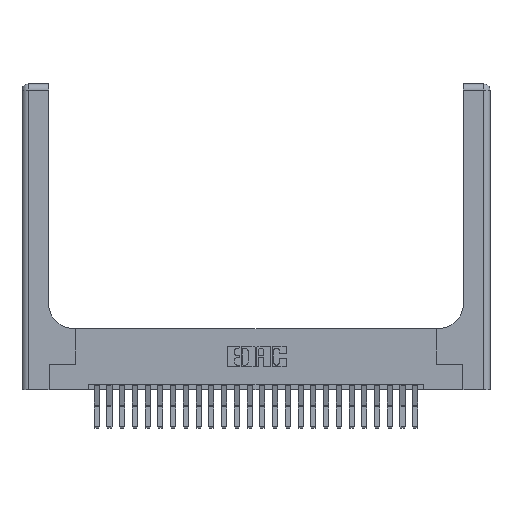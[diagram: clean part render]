
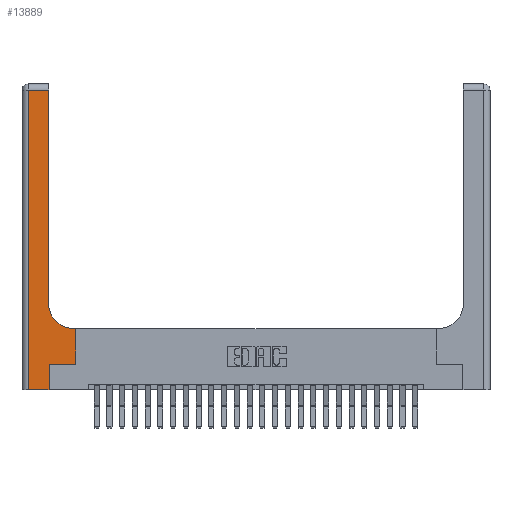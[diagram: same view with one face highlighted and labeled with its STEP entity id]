
A CAD part, top view. The second image highlights one B-rep face of the part: STEP entity #13889.
In plain terms, the highlighted planar face has unit normal (0, 0, 1).
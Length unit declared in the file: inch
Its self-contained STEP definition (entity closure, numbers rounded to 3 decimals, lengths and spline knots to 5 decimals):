
#484 = CARTESIAN_POINT ( 'NONE',  ( 0.51, 0.6, 0.37 ) ) ;
#2607 = VERTEX_POINT ( 'NONE', #21741 ) ;
#2796 = EDGE_CURVE ( 'NONE', #6051, #24206, #3019, .T. ) ;
#3019 = LINE ( 'NONE', #10699, #13411 ) ;
#3045 = VERTEX_POINT ( 'NONE', #20966 ) ;
#3153 = EDGE_CURVE ( 'NONE', #7943, #16102, #13583, .T. ) ;
#3191 = LINE ( 'NONE', #21906, #19430 ) ;
#3268 = PLANE ( 'NONE',  #17568 ) ;
#3340 = CARTESIAN_POINT ( 'NONE',  ( 0.06, 2.94, 0.37 ) ) ;
#3847 = VECTOR ( 'NONE', #20916, 39.37008 ) ;
#4181 = ORIENTED_EDGE ( 'NONE', *, *, #2796, .T. ) ;
#4547 = VERTEX_POINT ( 'NONE', #23224 ) ;
#4980 = VECTOR ( 'NONE', #13824, 39.37008 ) ;
#4985 = VECTOR ( 'NONE', #20823, 39.37008 ) ;
#5691 = EDGE_CURVE ( 'NONE', #17045, #9990, #9765, .T. ) ;
#5738 = CARTESIAN_POINT ( 'NONE',  ( 0.26, 0.6, 0.37 ) ) ;
#5907 = DIRECTION ( 'NONE',  ( -1., 0., 0. ) ) ;
#5972 = EDGE_CURVE ( 'NONE', #9990, #2607, #17877, .T. ) ;
#6051 = VERTEX_POINT ( 'NONE', #3340 ) ;
#6057 = DIRECTION ( 'NONE',  ( 0., 1., 0. ) ) ;
#6106 = EDGE_CURVE ( 'NONE', #16102, #17045, #7473, .T. ) ;
#6836 = ORIENTED_EDGE ( 'NONE', *, *, #21724, .T. ) ;
#7473 = LINE ( 'NONE', #18917, #3847 ) ;
#7943 = VERTEX_POINT ( 'NONE', #23792 ) ;
#8121 = ORIENTED_EDGE ( 'NONE', *, *, #19393, .T. ) ;
#8127 = ORIENTED_EDGE ( 'NONE', *, *, #21030, .T. ) ;
#8785 = FACE_OUTER_BOUND ( 'NONE', #21935, .T. ) ;
#8973 = CARTESIAN_POINT ( 'NONE',  ( 0.528, 0.25, 0.37 ) ) ;
#9025 = VECTOR ( 'NONE', #12688, 39.37008 ) ;
#9040 = DIRECTION ( 'NONE',  ( -1., 0., 0. ) ) ;
#9256 = CARTESIAN_POINT ( 'NONE',  ( 0.528, 0.6, 0.37 ) ) ;
#9765 = LINE ( 'NONE', #5738, #4985 ) ;
#9968 = ORIENTED_EDGE ( 'NONE', *, *, #5972, .T. ) ;
#9990 = VERTEX_POINT ( 'NONE', #484 ) ;
#10212 = LINE ( 'NONE', #17760, #21886 ) ;
#10324 = CARTESIAN_POINT ( 'NONE',  ( 0.06, 0., 0.37 ) ) ;
#10699 = CARTESIAN_POINT ( 'NONE',  ( 0.06, 3., 0.37 ) ) ;
#11335 = LINE ( 'NONE', #24800, #16090 ) ;
#12688 = DIRECTION ( 'NONE',  ( 1., 0., 0. ) ) ;
#13411 = VECTOR ( 'NONE', #20350, 39.37008 ) ;
#13583 = LINE ( 'NONE', #13706, #4980 ) ;
#13706 = CARTESIAN_POINT ( 'NONE',  ( 0.265, 0.25, 0.37 ) ) ;
#13824 = DIRECTION ( 'NONE',  ( 1., 0., 0. ) ) ;
#13889 = ADVANCED_FACE ( 'NONE', ( #8785 ), #3268, .F. ) ;
#14347 = ORIENTED_EDGE ( 'NONE', *, *, #3153, .T. ) ;
#14576 = CARTESIAN_POINT ( 'NONE',  ( 0., 0., 0.37 ) ) ;
#14847 = EDGE_CURVE ( 'NONE', #3045, #6051, #11335, .T. ) ;
#16090 = VECTOR ( 'NONE', #5907, 39.37008 ) ;
#16102 = VERTEX_POINT ( 'NONE', #8973 ) ;
#16276 = DIRECTION ( 'NONE',  ( 0., 1., 0. ) ) ;
#16551 = ORIENTED_EDGE ( 'NONE', *, *, #5691, .T. ) ;
#16680 = DIRECTION ( 'NONE',  ( 1., 0., 0. ) ) ;
#17045 = VERTEX_POINT ( 'NONE', #9256 ) ;
#17568 = AXIS2_PLACEMENT_3D ( 'NONE', #18598, #24390, #9040 ) ;
#17760 = CARTESIAN_POINT ( 'NONE',  ( 0.26, 3., 0.37 ) ) ;
#17877 = CIRCLE ( 'NONE', #21072, 0.25 ) ;
#18091 = LINE ( 'NONE', #14576, #9025 ) ;
#18181 = CARTESIAN_POINT ( 'NONE',  ( 0.51, 0.85, 0.37 ) ) ;
#18598 = CARTESIAN_POINT ( 'NONE',  ( 0., 3., 0.37 ) ) ;
#18917 = CARTESIAN_POINT ( 'NONE',  ( 0.528, 0.25, 0.37 ) ) ;
#19393 = EDGE_CURVE ( 'NONE', #4547, #7943, #3191, .T. ) ;
#19430 = VECTOR ( 'NONE', #16276, 39.37008 ) ;
#20350 = DIRECTION ( 'NONE',  ( 0., -1., 0. ) ) ;
#20823 = DIRECTION ( 'NONE',  ( -1., 0., 0. ) ) ;
#20916 = DIRECTION ( 'NONE',  ( 0., 1., 0. ) ) ;
#20966 = CARTESIAN_POINT ( 'NONE',  ( 0.26, 2.94, 0.37 ) ) ;
#21030 = EDGE_CURVE ( 'NONE', #2607, #3045, #10212, .T. ) ;
#21072 = AXIS2_PLACEMENT_3D ( 'NONE', #18181, #22439, #16680 ) ;
#21724 = EDGE_CURVE ( 'NONE', #24206, #4547, #18091, .T. ) ;
#21741 = CARTESIAN_POINT ( 'NONE',  ( 0.26, 0.85, 0.37 ) ) ;
#21886 = VECTOR ( 'NONE', #6057, 39.37008 ) ;
#21906 = CARTESIAN_POINT ( 'NONE',  ( 0.265, 0., 0.37 ) ) ;
#21935 = EDGE_LOOP ( 'NONE', ( #8127, #23402, #4181, #6836, #8121, #14347, #22312, #16551, #9968 ) ) ;
#22312 = ORIENTED_EDGE ( 'NONE', *, *, #6106, .T. ) ;
#22439 = DIRECTION ( 'NONE',  ( 0., 0., -1. ) ) ;
#23224 = CARTESIAN_POINT ( 'NONE',  ( 0.265, 0., 0.37 ) ) ;
#23402 = ORIENTED_EDGE ( 'NONE', *, *, #14847, .T. ) ;
#23792 = CARTESIAN_POINT ( 'NONE',  ( 0.265, 0.25, 0.37 ) ) ;
#24206 = VERTEX_POINT ( 'NONE', #10324 ) ;
#24390 = DIRECTION ( 'NONE',  ( 0., 0., -1. ) ) ;
#24800 = CARTESIAN_POINT ( 'NONE',  ( 0., 2.94, 0.37 ) ) ;
